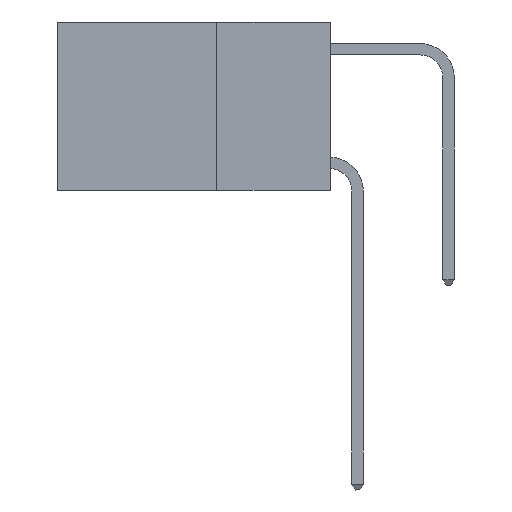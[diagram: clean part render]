
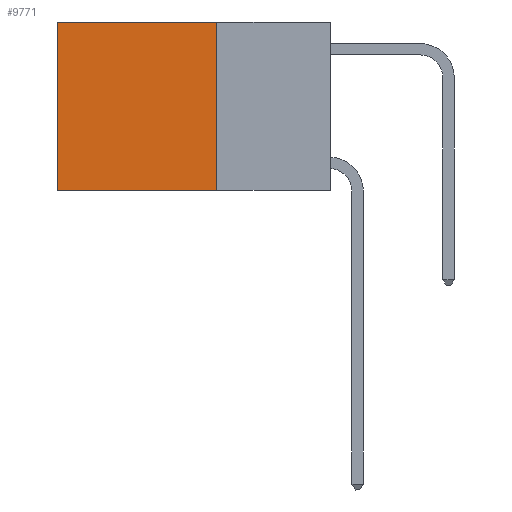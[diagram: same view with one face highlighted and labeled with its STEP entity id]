
A CAD part, left-side view. The second image highlights one B-rep face of the part: STEP entity #9771.
In plain terms, the highlighted planar face has unit normal (-1, 0, 0).
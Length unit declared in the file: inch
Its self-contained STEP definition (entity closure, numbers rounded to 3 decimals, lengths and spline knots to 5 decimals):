
#449 = DIRECTION ( 'NONE',  ( 0., 1., 0. ) ) ;
#577 = DIRECTION ( 'NONE',  ( 1., 0., 0. ) ) ;
#761 = VERTEX_POINT ( 'NONE', #7533 ) ;
#866 = LINE ( 'NONE', #1710, #6878 ) ;
#1475 = VECTOR ( 'NONE', #5086, 39.37008 ) ;
#1710 = CARTESIAN_POINT ( 'NONE',  ( 0.2625, 0.25, 0. ) ) ;
#2230 = CARTESIAN_POINT ( 'NONE',  ( 0.2625, 0.25, 0. ) ) ;
#2413 = CARTESIAN_POINT ( 'NONE',  ( 0.2625, 0.6, 0. ) ) ;
#2463 = PLANE ( 'NONE',  #3705 ) ;
#3045 = VERTEX_POINT ( 'NONE', #7426 ) ;
#3108 = VECTOR ( 'NONE', #449, 39.37008 ) ;
#3271 = CARTESIAN_POINT ( 'NONE',  ( 0.2625, 0.25, -0.37 ) ) ;
#3303 = LINE ( 'NONE', #10238, #3559 ) ;
#3559 = VECTOR ( 'NONE', #6870, 39.37008 ) ;
#3705 = AXIS2_PLACEMENT_3D ( 'NONE', #2230, #577, #11204 ) ;
#4292 = ORIENTED_EDGE ( 'NONE', *, *, #10706, .F. ) ;
#4480 = EDGE_CURVE ( 'NONE', #761, #9192, #7815, .T. ) ;
#5077 = ORIENTED_EDGE ( 'NONE', *, *, #7197, .T. ) ;
#5086 = DIRECTION ( 'NONE',  ( 0., 0., -1. ) ) ;
#5668 = EDGE_LOOP ( 'NONE', ( #5077, #4292, #6577, #8484 ) ) ;
#5787 = VERTEX_POINT ( 'NONE', #3271 ) ;
#6577 = ORIENTED_EDGE ( 'NONE', *, *, #8740, .F. ) ;
#6840 = LINE ( 'NONE', #2413, #1475 ) ;
#6870 = DIRECTION ( 'NONE',  ( 0., 1., 0. ) ) ;
#6878 = VECTOR ( 'NONE', #9893, 39.37008 ) ;
#7197 = EDGE_CURVE ( 'NONE', #9192, #3045, #6840, .T. ) ;
#7426 = CARTESIAN_POINT ( 'NONE',  ( 0.2625, 0.6, -0.37 ) ) ;
#7533 = CARTESIAN_POINT ( 'NONE',  ( 0.2625, 0.25, 0. ) ) ;
#7815 = LINE ( 'NONE', #9452, #3108 ) ;
#8484 = ORIENTED_EDGE ( 'NONE', *, *, #4480, .T. ) ;
#8740 = EDGE_CURVE ( 'NONE', #761, #5787, #866, .T. ) ;
#9192 = VERTEX_POINT ( 'NONE', #9368 ) ;
#9368 = CARTESIAN_POINT ( 'NONE',  ( 0.2625, 0.6, 0. ) ) ;
#9452 = CARTESIAN_POINT ( 'NONE',  ( 0.2625, 0.25, 0. ) ) ;
#9771 = ADVANCED_FACE ( 'NONE', ( #11432 ), #2463, .F. ) ;
#9893 = DIRECTION ( 'NONE',  ( 0., 0., -1. ) ) ;
#10238 = CARTESIAN_POINT ( 'NONE',  ( 0.2625, 0.25, -0.37 ) ) ;
#10706 = EDGE_CURVE ( 'NONE', #5787, #3045, #3303, .T. ) ;
#11204 = DIRECTION ( 'NONE',  ( 0., 0., -1. ) ) ;
#11432 = FACE_OUTER_BOUND ( 'NONE', #5668, .T. ) ;
